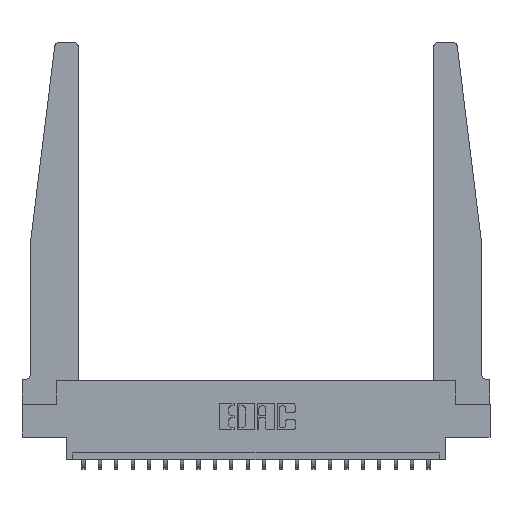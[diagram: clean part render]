
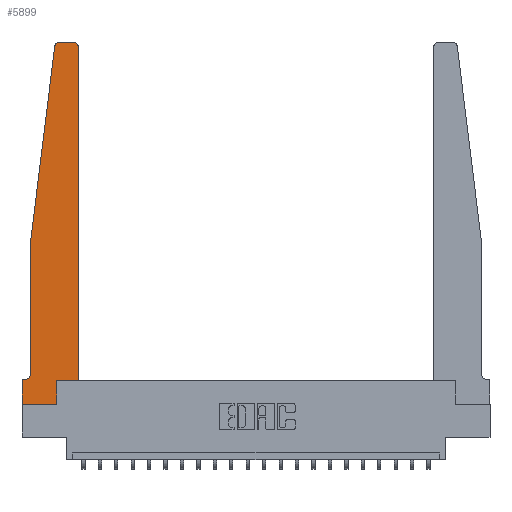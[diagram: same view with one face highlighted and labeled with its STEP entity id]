
A CAD part, top view. The second image highlights one B-rep face of the part: STEP entity #5899.
In plain terms, the highlighted planar face has unit normal (0, 0, 1).
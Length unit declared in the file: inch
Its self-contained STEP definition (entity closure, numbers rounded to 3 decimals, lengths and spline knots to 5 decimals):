
#121 = CARTESIAN_POINT ( 'NONE',  ( 0.065, 0.2375, 0.37 ) ) ;
#575 = CARTESIAN_POINT ( 'NONE',  ( 0.015, 0.2375, 0.37 ) ) ;
#786 = EDGE_CURVE ( 'NONE', #3452, #18596, #10483, .T. ) ;
#1197 = LINE ( 'NONE', #3064, #6654 ) ;
#1335 = VERTEX_POINT ( 'NONE', #6928 ) ;
#1443 = CARTESIAN_POINT ( 'NONE',  ( 0.065, 1.25, 0.37 ) ) ;
#1870 = VERTEX_POINT ( 'NONE', #5036 ) ;
#2187 = ORIENTED_EDGE ( 'NONE', *, *, #786, .T. ) ;
#2669 = VERTEX_POINT ( 'NONE', #19165 ) ;
#3064 = CARTESIAN_POINT ( 'NONE',  ( 0.25, 2.75, 0.37 ) ) ;
#3245 = LINE ( 'NONE', #18105, #4604 ) ;
#3259 = DIRECTION ( 'NONE',  ( 1., 0., 0. ) ) ;
#3321 = VERTEX_POINT ( 'NONE', #4461 ) ;
#3452 = VERTEX_POINT ( 'NONE', #5454 ) ;
#3740 = VECTOR ( 'NONE', #6030, 39.37008 ) ;
#3914 = VERTEX_POINT ( 'NONE', #14007 ) ;
#3948 = LINE ( 'NONE', #12623, #7387 ) ;
#4209 = VERTEX_POINT ( 'NONE', #121 ) ;
#4229 = ORIENTED_EDGE ( 'NONE', *, *, #5210, .T. ) ;
#4461 = CARTESIAN_POINT ( 'NONE',  ( 0., 0.1875, 0.37 ) ) ;
#4475 = VECTOR ( 'NONE', #7906, 39.37008 ) ;
#4604 = VECTOR ( 'NONE', #6518, 39.37008 ) ;
#4744 = CARTESIAN_POINT ( 'NONE',  ( 0.24675, 2.72367, 0.37 ) ) ;
#4857 = VERTEX_POINT ( 'NONE', #11044 ) ;
#5005 = PLANE ( 'NONE',  #19228 ) ;
#5036 = CARTESIAN_POINT ( 'NONE',  ( 0.27653, 2.75, 0.37 ) ) ;
#5210 = EDGE_CURVE ( 'NONE', #1335, #4209, #6023, .T. ) ;
#5325 = EDGE_CURVE ( 'NONE', #18596, #14551, #17212, .T. ) ;
#5454 = CARTESIAN_POINT ( 'NONE',  ( 0., 0., 0.37 ) ) ;
#5654 = CIRCLE ( 'NONE', #18332, 0.05 ) ;
#5666 = EDGE_CURVE ( 'NONE', #3914, #3321, #9196, .T. ) ;
#5833 = CARTESIAN_POINT ( 'NONE',  ( 0.395, 2.72, 0.37 ) ) ;
#5867 = CIRCLE ( 'NONE', #15738, 0.03 ) ;
#5899 = ADVANCED_FACE ( 'NONE', ( #13027 ), #5005, .T. ) ;
#6023 = LINE ( 'NONE', #10463, #18157 ) ;
#6030 = DIRECTION ( 'NONE',  ( 0., 1., 0. ) ) ;
#6518 = DIRECTION ( 'NONE',  ( 0., -1., 0. ) ) ;
#6654 = VECTOR ( 'NONE', #8009, 39.37008 ) ;
#6681 = CARTESIAN_POINT ( 'NONE',  ( 0.2605, 0.18, 0.37 ) ) ;
#6928 = CARTESIAN_POINT ( 'NONE',  ( 0.065, 1.25, 0.37 ) ) ;
#7299 = CARTESIAN_POINT ( 'NONE',  ( 0.27653, 2.72, 0.37 ) ) ;
#7387 = VECTOR ( 'NONE', #19481, 39.37008 ) ;
#7906 = DIRECTION ( 'NONE',  ( 0., 1., 0. ) ) ;
#8009 = DIRECTION ( 'NONE',  ( -1., 0., 0. ) ) ;
#8397 = EDGE_CURVE ( 'NONE', #4857, #10085, #19710, .T. ) ;
#8921 = DIRECTION ( 'NONE',  ( -1., 0., 0. ) ) ;
#8926 = DIRECTION ( 'NONE',  ( 0., -1., 0. ) ) ;
#9196 = LINE ( 'NONE', #15920, #18898 ) ;
#9446 = CARTESIAN_POINT ( 'NONE',  ( 0.425, 0.18, 0.37 ) ) ;
#9664 = ORIENTED_EDGE ( 'NONE', *, *, #5325, .T. ) ;
#10085 = VERTEX_POINT ( 'NONE', #17750 ) ;
#10215 = EDGE_CURVE ( 'NONE', #20867, #1335, #18177, .T. ) ;
#10277 = DIRECTION ( 'NONE',  ( 1., 0., 0. ) ) ;
#10463 = CARTESIAN_POINT ( 'NONE',  ( 0.065, 1.25, 0.37 ) ) ;
#10483 = LINE ( 'NONE', #15565, #16318 ) ;
#10595 = DIRECTION ( 'NONE',  ( 1., 0., 0. ) ) ;
#10627 = EDGE_CURVE ( 'NONE', #2669, #1870, #1197, .T. ) ;
#10778 = DIRECTION ( 'NONE',  ( 0., 0., 1. ) ) ;
#10861 = ORIENTED_EDGE ( 'NONE', *, *, #18472, .T. ) ;
#10934 = AXIS2_PLACEMENT_3D ( 'NONE', #7299, #20430, #10277 ) ;
#11044 = CARTESIAN_POINT ( 'NONE',  ( 0.425, 0.18, 0.37 ) ) ;
#12543 = DIRECTION ( 'NONE',  ( 1., 0., 0. ) ) ;
#12623 = CARTESIAN_POINT ( 'NONE',  ( 0.425, 0.18, 0.37 ) ) ;
#12800 = EDGE_CURVE ( 'NONE', #3321, #3452, #3245, .T. ) ;
#13027 = FACE_OUTER_BOUND ( 'NONE', #13993, .T. ) ;
#13248 = DIRECTION ( 'NONE',  ( 0., 0., 1. ) ) ;
#13410 = CIRCLE ( 'NONE', #10934, 0.03 ) ;
#13811 = CARTESIAN_POINT ( 'NONE',  ( 0.2605, 0.18, 0.37 ) ) ;
#13840 = EDGE_CURVE ( 'NONE', #4209, #3914, #5654, .T. ) ;
#13993 = EDGE_LOOP ( 'NONE', ( #21693, #19831, #16591, #4229, #20189, #18162, #16355, #2187, #9664, #21601, #17086, #10861 ) ) ;
#14007 = CARTESIAN_POINT ( 'NONE',  ( 0.015, 0.1875, 0.37 ) ) ;
#14476 = DIRECTION ( 'NONE',  ( -1., 0., 0. ) ) ;
#14542 = EDGE_CURVE ( 'NONE', #1870, #20867, #13410, .T. ) ;
#14551 = VERTEX_POINT ( 'NONE', #13811 ) ;
#14861 = DIRECTION ( 'NONE',  ( -0.122, -0.992, 0. ) ) ;
#15395 = CARTESIAN_POINT ( 'NONE',  ( 0.2605, 0., 0.37 ) ) ;
#15565 = CARTESIAN_POINT ( 'NONE',  ( 0., 0., 0.37 ) ) ;
#15738 = AXIS2_PLACEMENT_3D ( 'NONE', #5833, #10778, #12543 ) ;
#15920 = CARTESIAN_POINT ( 'NONE',  ( 0.065, 0.1875, 0.37 ) ) ;
#16318 = VECTOR ( 'NONE', #10595, 39.37008 ) ;
#16355 = ORIENTED_EDGE ( 'NONE', *, *, #12800, .T. ) ;
#16591 = ORIENTED_EDGE ( 'NONE', *, *, #10215, .T. ) ;
#17086 = ORIENTED_EDGE ( 'NONE', *, *, #8397, .T. ) ;
#17212 = LINE ( 'NONE', #6681, #3740 ) ;
#17750 = CARTESIAN_POINT ( 'NONE',  ( 0.425, 2.72, 0.37 ) ) ;
#17900 = CARTESIAN_POINT ( 'NONE',  ( 0., 0.1875, 0.37 ) ) ;
#18105 = CARTESIAN_POINT ( 'NONE',  ( 0., 0., 0.37 ) ) ;
#18157 = VECTOR ( 'NONE', #8926, 39.37008 ) ;
#18162 = ORIENTED_EDGE ( 'NONE', *, *, #5666, .T. ) ;
#18177 = LINE ( 'NONE', #1443, #20382 ) ;
#18332 = AXIS2_PLACEMENT_3D ( 'NONE', #575, #19399, #8921 ) ;
#18472 = EDGE_CURVE ( 'NONE', #10085, #2669, #5867, .T. ) ;
#18596 = VERTEX_POINT ( 'NONE', #15395 ) ;
#18898 = VECTOR ( 'NONE', #14476, 39.37008 ) ;
#19165 = CARTESIAN_POINT ( 'NONE',  ( 0.395, 2.75, 0.37 ) ) ;
#19228 = AXIS2_PLACEMENT_3D ( 'NONE', #17900, #13248, #3259 ) ;
#19399 = DIRECTION ( 'NONE',  ( 0., 0., -1. ) ) ;
#19481 = DIRECTION ( 'NONE',  ( 1., 0., 0. ) ) ;
#19710 = LINE ( 'NONE', #9446, #4475 ) ;
#19831 = ORIENTED_EDGE ( 'NONE', *, *, #14542, .T. ) ;
#20189 = ORIENTED_EDGE ( 'NONE', *, *, #13840, .T. ) ;
#20382 = VECTOR ( 'NONE', #14861, 39.37008 ) ;
#20430 = DIRECTION ( 'NONE',  ( 0., 0., 1. ) ) ;
#20867 = VERTEX_POINT ( 'NONE', #4744 ) ;
#21601 = ORIENTED_EDGE ( 'NONE', *, *, #21615, .T. ) ;
#21615 = EDGE_CURVE ( 'NONE', #14551, #4857, #3948, .T. ) ;
#21693 = ORIENTED_EDGE ( 'NONE', *, *, #10627, .T. ) ;
